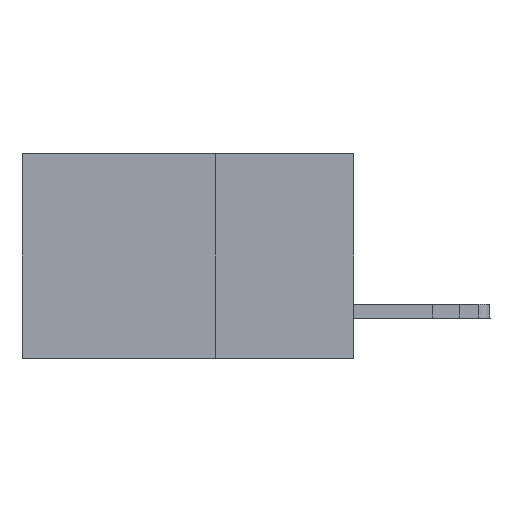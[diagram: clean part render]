
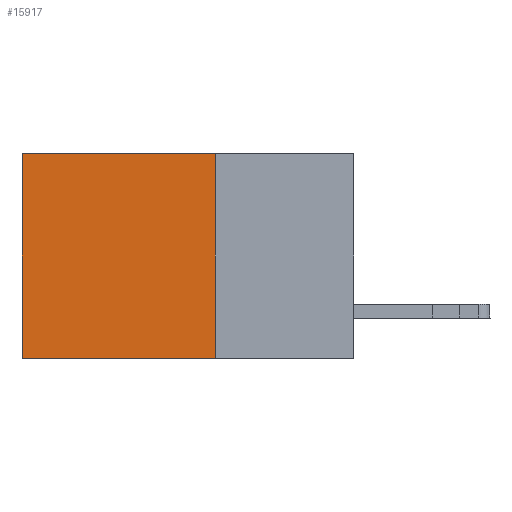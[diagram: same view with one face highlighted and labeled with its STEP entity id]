
A CAD part, left-side view. The second image highlights one B-rep face of the part: STEP entity #15917.
In plain terms, the highlighted planar face has unit normal (-1, 0, 0).
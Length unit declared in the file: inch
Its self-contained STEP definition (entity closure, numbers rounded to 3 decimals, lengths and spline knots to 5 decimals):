
#1380 = ORIENTED_EDGE ( 'NONE', *, *, #15829, .F. ) ;
#2033 = VERTEX_POINT ( 'NONE', #19998 ) ;
#2313 = VERTEX_POINT ( 'NONE', #9065 ) ;
#3192 = VECTOR ( 'NONE', #9888, 39.37008 ) ;
#3203 = VERTEX_POINT ( 'NONE', #13440 ) ;
#4057 = EDGE_CURVE ( 'NONE', #2313, #3203, #21437, .T. ) ;
#5526 = LINE ( 'NONE', #13909, #13995 ) ;
#5693 = CARTESIAN_POINT ( 'NONE',  ( 0.2875, 0.25, 0. ) ) ;
#7355 = EDGE_CURVE ( 'NONE', #2033, #9106, #12889, .T. ) ;
#7377 = DIRECTION ( 'NONE',  ( 0., 0., -1. ) ) ;
#7748 = ORIENTED_EDGE ( 'NONE', *, *, #7355, .F. ) ;
#8235 = VECTOR ( 'NONE', #20801, 39.37008 ) ;
#9029 = ORIENTED_EDGE ( 'NONE', *, *, #4057, .T. ) ;
#9065 = CARTESIAN_POINT ( 'NONE',  ( 0.2875, 0.25, 0. ) ) ;
#9106 = VERTEX_POINT ( 'NONE', #19124 ) ;
#9888 = DIRECTION ( 'NONE',  ( 0., 0., -1. ) ) ;
#10954 = CARTESIAN_POINT ( 'NONE',  ( 0.2875, 0.25, 0. ) ) ;
#11129 = AXIS2_PLACEMENT_3D ( 'NONE', #5693, #17396, #7377 ) ;
#11663 = LINE ( 'NONE', #19750, #3192 ) ;
#12419 = FACE_OUTER_BOUND ( 'NONE', #14715, .T. ) ;
#12888 = DIRECTION ( 'NONE',  ( 0., 1., 0. ) ) ;
#12889 = LINE ( 'NONE', #17729, #13410 ) ;
#13410 = VECTOR ( 'NONE', #12888, 39.37008 ) ;
#13440 = CARTESIAN_POINT ( 'NONE',  ( 0.2875, 0.6, 0. ) ) ;
#13909 = CARTESIAN_POINT ( 'NONE',  ( 0.2875, 0.25, 0. ) ) ;
#13995 = VECTOR ( 'NONE', #17134, 39.37008 ) ;
#14126 = PLANE ( 'NONE',  #11129 ) ;
#14715 = EDGE_LOOP ( 'NONE', ( #20051, #7748, #1380, #9029 ) ) ;
#15829 = EDGE_CURVE ( 'NONE', #2313, #2033, #5526, .T. ) ;
#15917 = ADVANCED_FACE ( 'NONE', ( #12419 ), #14126, .F. ) ;
#17134 = DIRECTION ( 'NONE',  ( 0., 0., -1. ) ) ;
#17396 = DIRECTION ( 'NONE',  ( 1., 0., 0. ) ) ;
#17729 = CARTESIAN_POINT ( 'NONE',  ( 0.2875, 0.25, -0.37 ) ) ;
#19124 = CARTESIAN_POINT ( 'NONE',  ( 0.2875, 0.6, -0.37 ) ) ;
#19750 = CARTESIAN_POINT ( 'NONE',  ( 0.2875, 0.6, 0. ) ) ;
#19998 = CARTESIAN_POINT ( 'NONE',  ( 0.2875, 0.25, -0.37 ) ) ;
#20051 = ORIENTED_EDGE ( 'NONE', *, *, #21256, .T. ) ;
#20801 = DIRECTION ( 'NONE',  ( 0., 1., 0. ) ) ;
#21256 = EDGE_CURVE ( 'NONE', #3203, #9106, #11663, .T. ) ;
#21437 = LINE ( 'NONE', #10954, #8235 ) ;
